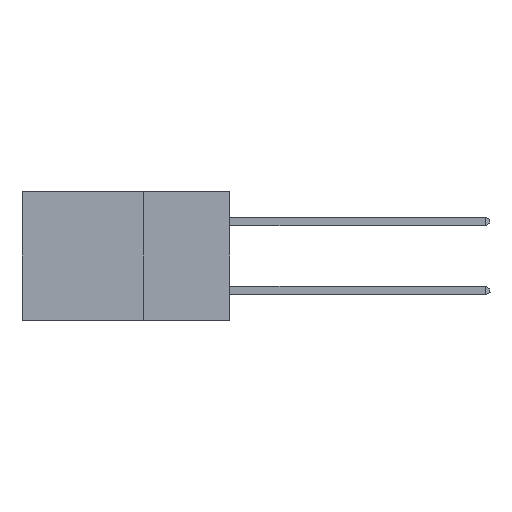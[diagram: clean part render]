
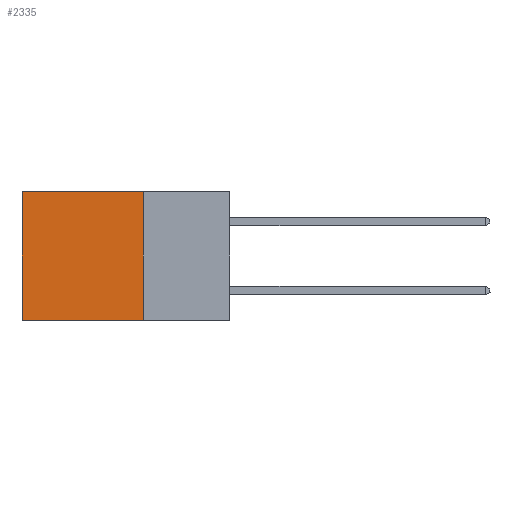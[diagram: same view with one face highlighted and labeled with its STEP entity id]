
A CAD part, left-side view. The second image highlights one B-rep face of the part: STEP entity #2335.
In plain terms, the highlighted planar face has unit normal (-1, 0, 0).
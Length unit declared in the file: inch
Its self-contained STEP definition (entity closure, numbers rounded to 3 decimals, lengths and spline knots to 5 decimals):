
#488 = VERTEX_POINT ( 'NONE', #8240 ) ;
#744 = VECTOR ( 'NONE', #7525, 39.37008 ) ;
#785 = LINE ( 'NONE', #11961, #6195 ) ;
#963 = LINE ( 'NONE', #12838, #4552 ) ;
#1988 = LINE ( 'NONE', #12234, #744 ) ;
#2335 = ADVANCED_FACE ( 'NONE', ( #14245 ), #10045, .F. ) ;
#3313 = CARTESIAN_POINT ( 'NONE',  ( 0.298, 0.25, 0. ) ) ;
#3682 = EDGE_CURVE ( 'NONE', #13551, #11951, #12168, .T. ) ;
#4005 = VERTEX_POINT ( 'NONE', #4400 ) ;
#4337 = DIRECTION ( 'NONE',  ( 1., 0., 0. ) ) ;
#4400 = CARTESIAN_POINT ( 'NONE',  ( 0.298, 0.25, 0. ) ) ;
#4552 = VECTOR ( 'NONE', #12887, 39.37008 ) ;
#5512 = DIRECTION ( 'NONE',  ( 0., 0., -1. ) ) ;
#6195 = VECTOR ( 'NONE', #12015, 39.37008 ) ;
#6895 = EDGE_CURVE ( 'NONE', #488, #11951, #785, .T. ) ;
#7525 = DIRECTION ( 'NONE',  ( 0., 1., 0. ) ) ;
#7804 = EDGE_LOOP ( 'NONE', ( #13854, #7894, #9057, #13096 ) ) ;
#7894 = ORIENTED_EDGE ( 'NONE', *, *, #6895, .F. ) ;
#8232 = EDGE_CURVE ( 'NONE', #4005, #13551, #1988, .T. ) ;
#8240 = CARTESIAN_POINT ( 'NONE',  ( 0.298, 0.25, -0.37 ) ) ;
#9057 = ORIENTED_EDGE ( 'NONE', *, *, #10714, .F. ) ;
#9149 = VECTOR ( 'NONE', #12946, 39.37008 ) ;
#9315 = CARTESIAN_POINT ( 'NONE',  ( 0.298, 0.6, 0. ) ) ;
#10045 = PLANE ( 'NONE',  #12633 ) ;
#10714 = EDGE_CURVE ( 'NONE', #4005, #488, #963, .T. ) ;
#10810 = CARTESIAN_POINT ( 'NONE',  ( 0.298, 0.6, 0. ) ) ;
#11152 = CARTESIAN_POINT ( 'NONE',  ( 0.298, 0.6, -0.37 ) ) ;
#11951 = VERTEX_POINT ( 'NONE', #11152 ) ;
#11961 = CARTESIAN_POINT ( 'NONE',  ( 0.298, 0.25, -0.37 ) ) ;
#12015 = DIRECTION ( 'NONE',  ( 0., 1., 0. ) ) ;
#12168 = LINE ( 'NONE', #10810, #9149 ) ;
#12234 = CARTESIAN_POINT ( 'NONE',  ( 0.298, 0.25, 0. ) ) ;
#12633 = AXIS2_PLACEMENT_3D ( 'NONE', #3313, #4337, #5512 ) ;
#12838 = CARTESIAN_POINT ( 'NONE',  ( 0.298, 0.25, 0. ) ) ;
#12887 = DIRECTION ( 'NONE',  ( 0., 0., -1. ) ) ;
#12946 = DIRECTION ( 'NONE',  ( 0., 0., -1. ) ) ;
#13096 = ORIENTED_EDGE ( 'NONE', *, *, #8232, .T. ) ;
#13551 = VERTEX_POINT ( 'NONE', #9315 ) ;
#13854 = ORIENTED_EDGE ( 'NONE', *, *, #3682, .T. ) ;
#14245 = FACE_OUTER_BOUND ( 'NONE', #7804, .T. ) ;
